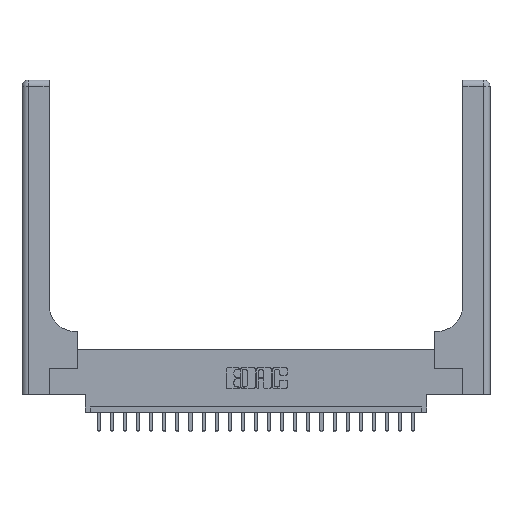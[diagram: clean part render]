
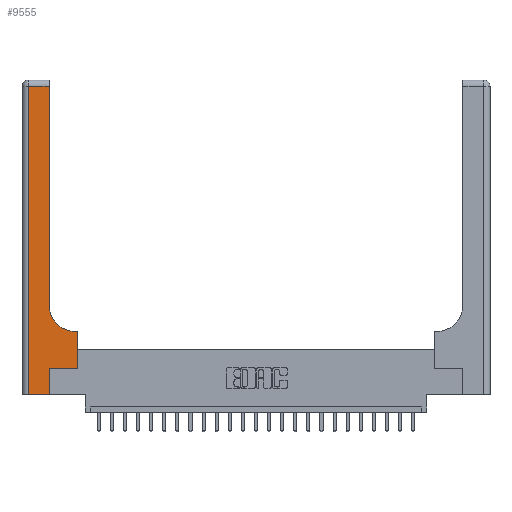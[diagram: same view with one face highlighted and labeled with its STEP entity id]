
A CAD part, top view. The second image highlights one B-rep face of the part: STEP entity #9555.
In plain terms, the highlighted planar face has unit normal (0, 0, 1).
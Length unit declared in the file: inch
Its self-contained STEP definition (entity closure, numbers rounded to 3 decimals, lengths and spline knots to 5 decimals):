
#841 = LINE ( 'NONE', #21332, #20219 ) ;
#933 = VERTEX_POINT ( 'NONE', #10474 ) ;
#2001 = AXIS2_PLACEMENT_3D ( 'NONE', #18168, #16161, #21535 ) ;
#2362 = EDGE_CURVE ( 'NONE', #3476, #20037, #18955, .T. ) ;
#3071 = VERTEX_POINT ( 'NONE', #23066 ) ;
#3124 = VERTEX_POINT ( 'NONE', #18830 ) ;
#3476 = VERTEX_POINT ( 'NONE', #3778 ) ;
#3765 = VECTOR ( 'NONE', #6376, 39.37008 ) ;
#3778 = CARTESIAN_POINT ( 'NONE',  ( 0.06, 2.94, 0.37 ) ) ;
#4598 = VERTEX_POINT ( 'NONE', #16845 ) ;
#4675 = PLANE ( 'NONE',  #13421 ) ;
#4810 = CARTESIAN_POINT ( 'NONE',  ( 0.26, 2.94, 0.37 ) ) ;
#4823 = CARTESIAN_POINT ( 'NONE',  ( 0., 0., 0.37 ) ) ;
#5450 = VECTOR ( 'NONE', #14695, 39.37008 ) ;
#6052 = VECTOR ( 'NONE', #22339, 39.37008 ) ;
#6128 = ORIENTED_EDGE ( 'NONE', *, *, #13694, .T. ) ;
#6256 = FACE_OUTER_BOUND ( 'NONE', #16876, .T. ) ;
#6376 = DIRECTION ( 'NONE',  ( 0., 1., 0. ) ) ;
#6720 = DIRECTION ( 'NONE',  ( 1., 0., 0. ) ) ;
#7077 = ORIENTED_EDGE ( 'NONE', *, *, #14917, .T. ) ;
#7179 = LINE ( 'NONE', #12985, #5450 ) ;
#7899 = LINE ( 'NONE', #20961, #11494 ) ;
#7916 = LINE ( 'NONE', #11978, #17142 ) ;
#7928 = DIRECTION ( 'NONE',  ( 0., -1., 0. ) ) ;
#8125 = CARTESIAN_POINT ( 'NONE',  ( 0.26, 3., 0.37 ) ) ;
#8533 = ORIENTED_EDGE ( 'NONE', *, *, #23128, .T. ) ;
#8595 = LINE ( 'NONE', #8125, #3765 ) ;
#8873 = ORIENTED_EDGE ( 'NONE', *, *, #12941, .T. ) ;
#8882 = CARTESIAN_POINT ( 'NONE',  ( 0.06, 0., 0.37 ) ) ;
#9555 = ADVANCED_FACE ( 'NONE', ( #6256 ), #4675, .F. ) ;
#9954 = VERTEX_POINT ( 'NONE', #10024 ) ;
#10024 = CARTESIAN_POINT ( 'NONE',  ( 0.26, 0.85, 0.37 ) ) ;
#10343 = DIRECTION ( 'NONE',  ( -1., 0., 0. ) ) ;
#10474 = CARTESIAN_POINT ( 'NONE',  ( 0.528, 0.25, 0.37 ) ) ;
#10814 = VECTOR ( 'NONE', #7928, 39.37008 ) ;
#11059 = DIRECTION ( 'NONE',  ( -1., 0., 0. ) ) ;
#11494 = VECTOR ( 'NONE', #12160, 39.37008 ) ;
#11542 = CARTESIAN_POINT ( 'NONE',  ( 0.51, 0.6, 0.37 ) ) ;
#11636 = CIRCLE ( 'NONE', #2001, 0.25 ) ;
#11978 = CARTESIAN_POINT ( 'NONE',  ( 0.265, 0., 0.37 ) ) ;
#11990 = ORIENTED_EDGE ( 'NONE', *, *, #2362, .T. ) ;
#12160 = DIRECTION ( 'NONE',  ( 1., 0., 0. ) ) ;
#12941 = EDGE_CURVE ( 'NONE', #933, #4598, #21801, .T. ) ;
#12985 = CARTESIAN_POINT ( 'NONE',  ( 0.26, 0.6, 0.37 ) ) ;
#13421 = AXIS2_PLACEMENT_3D ( 'NONE', #20941, #15496, #10343 ) ;
#13445 = EDGE_CURVE ( 'NONE', #9954, #20962, #8595, .T. ) ;
#13579 = LINE ( 'NONE', #4823, #16061 ) ;
#13694 = EDGE_CURVE ( 'NONE', #4598, #14020, #7179, .T. ) ;
#13848 = DIRECTION ( 'NONE',  ( 0., 1., 0. ) ) ;
#14020 = VERTEX_POINT ( 'NONE', #11542 ) ;
#14440 = ORIENTED_EDGE ( 'NONE', *, *, #21237, .T. ) ;
#14586 = ORIENTED_EDGE ( 'NONE', *, *, #17601, .T. ) ;
#14695 = DIRECTION ( 'NONE',  ( -1., 0., 0. ) ) ;
#14917 = EDGE_CURVE ( 'NONE', #20037, #3124, #13579, .T. ) ;
#14957 = ORIENTED_EDGE ( 'NONE', *, *, #17790, .T. ) ;
#15496 = DIRECTION ( 'NONE',  ( 0., 0., -1. ) ) ;
#16061 = VECTOR ( 'NONE', #6720, 39.37008 ) ;
#16161 = DIRECTION ( 'NONE',  ( 0., 0., -1. ) ) ;
#16845 = CARTESIAN_POINT ( 'NONE',  ( 0.528, 0.6, 0.37 ) ) ;
#16876 = EDGE_LOOP ( 'NONE', ( #20808, #14957, #11990, #7077, #8533, #14586, #8873, #6128, #14440 ) ) ;
#17142 = VECTOR ( 'NONE', #13848, 39.37008 ) ;
#17601 = EDGE_CURVE ( 'NONE', #3071, #933, #7899, .T. ) ;
#17790 = EDGE_CURVE ( 'NONE', #20962, #3476, #841, .T. ) ;
#18168 = CARTESIAN_POINT ( 'NONE',  ( 0.51, 0.85, 0.37 ) ) ;
#18644 = CARTESIAN_POINT ( 'NONE',  ( 0.06, 3., 0.37 ) ) ;
#18830 = CARTESIAN_POINT ( 'NONE',  ( 0.265, 0., 0.37 ) ) ;
#18955 = LINE ( 'NONE', #18644, #10814 ) ;
#20037 = VERTEX_POINT ( 'NONE', #8882 ) ;
#20219 = VECTOR ( 'NONE', #11059, 39.37008 ) ;
#20808 = ORIENTED_EDGE ( 'NONE', *, *, #13445, .T. ) ;
#20941 = CARTESIAN_POINT ( 'NONE',  ( 0., 3., 0.37 ) ) ;
#20961 = CARTESIAN_POINT ( 'NONE',  ( 0.265, 0.25, 0.37 ) ) ;
#20962 = VERTEX_POINT ( 'NONE', #4810 ) ;
#21237 = EDGE_CURVE ( 'NONE', #14020, #9954, #11636, .T. ) ;
#21332 = CARTESIAN_POINT ( 'NONE',  ( 0., 2.94, 0.37 ) ) ;
#21535 = DIRECTION ( 'NONE',  ( 1., 0., 0. ) ) ;
#21801 = LINE ( 'NONE', #22420, #6052 ) ;
#22339 = DIRECTION ( 'NONE',  ( 0., 1., 0. ) ) ;
#22420 = CARTESIAN_POINT ( 'NONE',  ( 0.528, 0.25, 0.37 ) ) ;
#23066 = CARTESIAN_POINT ( 'NONE',  ( 0.265, 0.25, 0.37 ) ) ;
#23128 = EDGE_CURVE ( 'NONE', #3124, #3071, #7916, .T. ) ;
